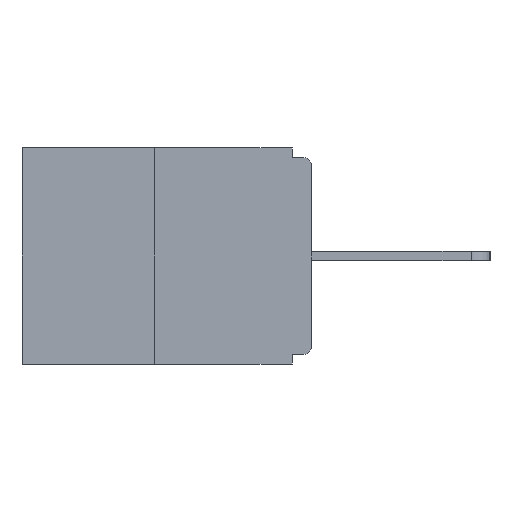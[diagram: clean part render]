
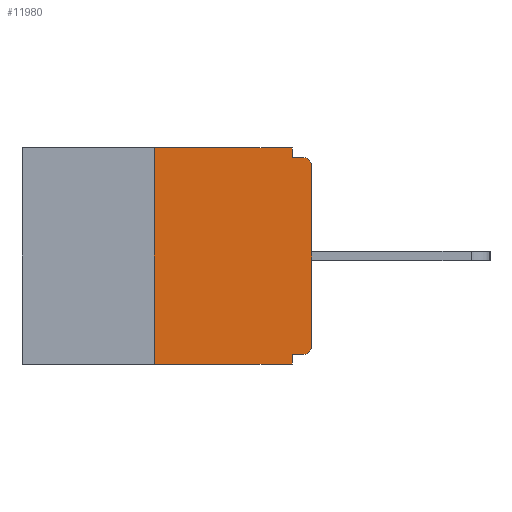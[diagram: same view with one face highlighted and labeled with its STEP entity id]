
A CAD part, left-side view. The second image highlights one B-rep face of the part: STEP entity #11980.
In plain terms, the highlighted planar face has unit normal (-1, 0, 0).
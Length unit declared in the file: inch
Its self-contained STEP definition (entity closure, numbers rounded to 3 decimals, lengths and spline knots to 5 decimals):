
#4 = CARTESIAN_POINT ( 'NONE',  ( 0., 0., 0. ) ) ;
#396 = CIRCLE ( 'NONE', #1236, 0.015 ) ;
#530 = VECTOR ( 'NONE', #15956, 39.37008 ) ;
#626 = VERTEX_POINT ( 'NONE', #3003 ) ;
#742 = EDGE_LOOP ( 'NONE', ( #6860, #6292, #15017, #13557, #8605, #11090, #6533, #7631, #9266, #7441 ) ) ;
#1236 = AXIS2_PLACEMENT_3D ( 'NONE', #9344, #1381, #10667 ) ;
#1381 = DIRECTION ( 'NONE',  ( -1., 0., 0. ) ) ;
#1454 = FACE_OUTER_BOUND ( 'NONE', #742, .T. ) ;
#1999 = VECTOR ( 'NONE', #13707, 39.37008 ) ;
#2414 = VERTEX_POINT ( 'NONE', #8219 ) ;
#2792 = PLANE ( 'NONE',  #10398 ) ;
#2973 = VERTEX_POINT ( 'NONE', #7690 ) ;
#3003 = CARTESIAN_POINT ( 'NONE',  ( 0., 0.25, 0. ) ) ;
#3640 = VECTOR ( 'NONE', #4100, 39.37008 ) ;
#3928 = LINE ( 'NONE', #15425, #7079 ) ;
#4100 = DIRECTION ( 'NONE',  ( 0., 0., -1. ) ) ;
#4158 = DIRECTION ( 'NONE',  ( 1., 0., 0. ) ) ;
#4654 = CARTESIAN_POINT ( 'NONE',  ( 0., 0., -0.03 ) ) ;
#4760 = EDGE_CURVE ( 'NONE', #12742, #7095, #15722, .T. ) ;
#5068 = DIRECTION ( 'NONE',  ( 0., -1., 0. ) ) ;
#5140 = EDGE_CURVE ( 'NONE', #16597, #13165, #12990, .T. ) ;
#5415 = LINE ( 'NONE', #4, #12048 ) ;
#5490 = EDGE_CURVE ( 'NONE', #7095, #2414, #14221, .T. ) ;
#5963 = VECTOR ( 'NONE', #5068, 39.37008 ) ;
#6292 = ORIENTED_EDGE ( 'NONE', *, *, #7075, .F. ) ;
#6533 = ORIENTED_EDGE ( 'NONE', *, *, #12400, .T. ) ;
#6690 = CARTESIAN_POINT ( 'NONE',  ( 0., 0.031, 0. ) ) ;
#6860 = ORIENTED_EDGE ( 'NONE', *, *, #9946, .F. ) ;
#7075 = EDGE_CURVE ( 'NONE', #8588, #626, #16283, .T. ) ;
#7079 = VECTOR ( 'NONE', #8820, 39.37008 ) ;
#7095 = VERTEX_POINT ( 'NONE', #13014 ) ;
#7244 = LINE ( 'NONE', #6690, #530 ) ;
#7347 = CARTESIAN_POINT ( 'NONE',  ( 0., 0.031, 0. ) ) ;
#7441 = ORIENTED_EDGE ( 'NONE', *, *, #16070, .F. ) ;
#7607 = DIRECTION ( 'NONE',  ( -1., 0., 0. ) ) ;
#7631 = ORIENTED_EDGE ( 'NONE', *, *, #9074, .T. ) ;
#7690 = CARTESIAN_POINT ( 'NONE',  ( 0., 0., -0.313 ) ) ;
#8147 = VERTEX_POINT ( 'NONE', #4654 ) ;
#8219 = CARTESIAN_POINT ( 'NONE',  ( 0., 0.031, -0.343 ) ) ;
#8588 = VERTEX_POINT ( 'NONE', #9492 ) ;
#8605 = ORIENTED_EDGE ( 'NONE', *, *, #4760, .F. ) ;
#8712 = CARTESIAN_POINT ( 'NONE',  ( 0., 0.015, -0.328 ) ) ;
#8820 = DIRECTION ( 'NONE',  ( 0., -1., 0. ) ) ;
#9074 = EDGE_CURVE ( 'NONE', #8147, #13165, #396, .T. ) ;
#9151 = VECTOR ( 'NONE', #9756, 39.37008 ) ;
#9266 = ORIENTED_EDGE ( 'NONE', *, *, #5140, .F. ) ;
#9344 = CARTESIAN_POINT ( 'NONE',  ( 0., 0.015, -0.03 ) ) ;
#9492 = CARTESIAN_POINT ( 'NONE',  ( 0., 0.25, -0.343 ) ) ;
#9618 = VECTOR ( 'NONE', #12736, 39.37008 ) ;
#9756 = DIRECTION ( 'NONE',  ( 0., -1., 0. ) ) ;
#9849 = AXIS2_PLACEMENT_3D ( 'NONE', #15527, #7607, #16868 ) ;
#9946 = EDGE_CURVE ( 'NONE', #626, #15853, #3928, .T. ) ;
#10398 = AXIS2_PLACEMENT_3D ( 'NONE', #12096, #4158, #13412 ) ;
#10485 = CIRCLE ( 'NONE', #9849, 0.015 ) ;
#10546 = CARTESIAN_POINT ( 'NONE',  ( 0., 0., -0.015 ) ) ;
#10667 = DIRECTION ( 'NONE',  ( 0., 0., -1. ) ) ;
#11090 = ORIENTED_EDGE ( 'NONE', *, *, #11699, .T. ) ;
#11408 = CARTESIAN_POINT ( 'NONE',  ( 0., 0.25, 0. ) ) ;
#11699 = EDGE_CURVE ( 'NONE', #12742, #2973, #10485, .T. ) ;
#11980 = ADVANCED_FACE ( 'NONE', ( #1454 ), #2792, .F. ) ;
#12048 = VECTOR ( 'NONE', #15955, 39.37008 ) ;
#12096 = CARTESIAN_POINT ( 'NONE',  ( 0., 0.46, 0. ) ) ;
#12144 = EDGE_CURVE ( 'NONE', #8588, #2414, #13084, .T. ) ;
#12386 = CARTESIAN_POINT ( 'NONE',  ( 0., 0.46, -0.343 ) ) ;
#12400 = EDGE_CURVE ( 'NONE', #2973, #8147, #5415, .T. ) ;
#12736 = DIRECTION ( 'NONE',  ( 0., 0., 1. ) ) ;
#12742 = VERTEX_POINT ( 'NONE', #8712 ) ;
#12990 = LINE ( 'NONE', #10546, #5963 ) ;
#13014 = CARTESIAN_POINT ( 'NONE',  ( 0., 0.031, -0.328 ) ) ;
#13019 = CARTESIAN_POINT ( 'NONE',  ( 0., 0.031, -0.015 ) ) ;
#13084 = LINE ( 'NONE', #12386, #9151 ) ;
#13165 = VERTEX_POINT ( 'NONE', #13607 ) ;
#13302 = CARTESIAN_POINT ( 'NONE',  ( 0., 0.031, -0.343 ) ) ;
#13412 = DIRECTION ( 'NONE',  ( 0., 0., -1. ) ) ;
#13557 = ORIENTED_EDGE ( 'NONE', *, *, #5490, .F. ) ;
#13607 = CARTESIAN_POINT ( 'NONE',  ( 0., 0.015, -0.015 ) ) ;
#13707 = DIRECTION ( 'NONE',  ( 0., 1., 0. ) ) ;
#13726 = CARTESIAN_POINT ( 'NONE',  ( 0., 0., -0.328 ) ) ;
#14221 = LINE ( 'NONE', #13302, #3640 ) ;
#15017 = ORIENTED_EDGE ( 'NONE', *, *, #12144, .T. ) ;
#15425 = CARTESIAN_POINT ( 'NONE',  ( 0., 0.46, 0. ) ) ;
#15527 = CARTESIAN_POINT ( 'NONE',  ( 0., 0.015, -0.313 ) ) ;
#15722 = LINE ( 'NONE', #13726, #1999 ) ;
#15853 = VERTEX_POINT ( 'NONE', #7347 ) ;
#15955 = DIRECTION ( 'NONE',  ( 0., 0., 1. ) ) ;
#15956 = DIRECTION ( 'NONE',  ( 0., 0., -1. ) ) ;
#16070 = EDGE_CURVE ( 'NONE', #15853, #16597, #7244, .T. ) ;
#16283 = LINE ( 'NONE', #11408, #9618 ) ;
#16597 = VERTEX_POINT ( 'NONE', #13019 ) ;
#16868 = DIRECTION ( 'NONE',  ( 0., 0., -1. ) ) ;
